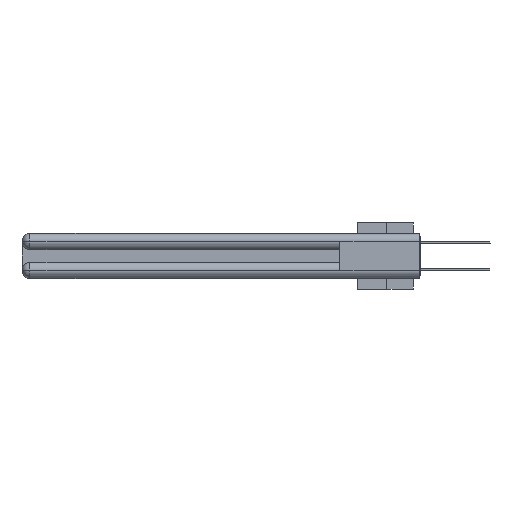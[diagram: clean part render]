
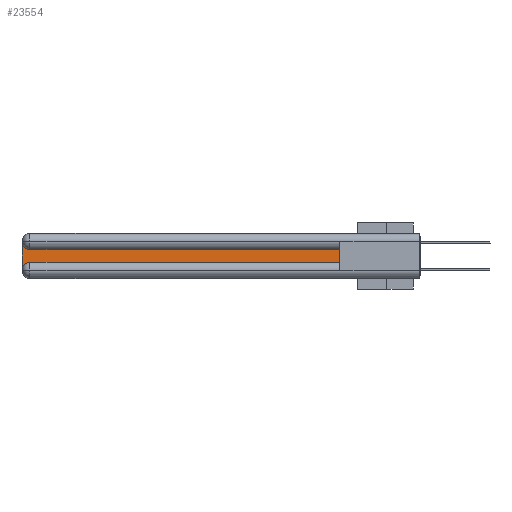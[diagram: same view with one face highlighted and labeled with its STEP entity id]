
A CAD part, left-side view. The second image highlights one B-rep face of the part: STEP entity #23554.
In plain terms, the highlighted planar face has unit normal (-1, 0, 0).
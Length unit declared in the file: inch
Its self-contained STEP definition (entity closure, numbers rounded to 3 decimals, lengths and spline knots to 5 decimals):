
#914 = CARTESIAN_POINT ( 'NONE',  ( 0.075, 2.94, -0.2775 ) ) ;
#1142 = DIRECTION ( 'NONE',  ( 1., 0., 0. ) ) ;
#2474 = VERTEX_POINT ( 'NONE', #17061 ) ;
#2644 = EDGE_CURVE ( 'NONE', #6175, #24458, #26580, .T. ) ;
#3265 = DIRECTION ( 'NONE',  ( 1., 0., 0. ) ) ;
#3273 = DIRECTION ( 'NONE',  ( 0., 0., -1. ) ) ;
#4350 = ORIENTED_EDGE ( 'NONE', *, *, #5753, .T. ) ;
#4694 = CARTESIAN_POINT ( 'NONE',  ( 0.075, 0.6, -0.1225 ) ) ;
#5704 = EDGE_CURVE ( 'NONE', #15519, #9257, #32199, .T. ) ;
#5753 = EDGE_CURVE ( 'NONE', #24458, #15519, #16304, .T. ) ;
#6175 = VERTEX_POINT ( 'NONE', #34233 ) ;
#7078 = EDGE_LOOP ( 'NONE', ( #9344, #14548, #9575, #26792, #8776, #4350 ) ) ;
#8245 = CARTESIAN_POINT ( 'NONE',  ( 0.075, 0.6, -0.2175 ) ) ;
#8471 = FACE_OUTER_BOUND ( 'NONE', #7078, .T. ) ;
#8776 = ORIENTED_EDGE ( 'NONE', *, *, #2644, .T. ) ;
#9257 = VERTEX_POINT ( 'NONE', #30815 ) ;
#9344 = ORIENTED_EDGE ( 'NONE', *, *, #5704, .T. ) ;
#9575 = ORIENTED_EDGE ( 'NONE', *, *, #25790, .T. ) ;
#10048 = DIRECTION ( 'NONE',  ( 0., -1., 0. ) ) ;
#10957 = CIRCLE ( 'NONE', #33094, 0.06 ) ;
#11924 = DIRECTION ( 'NONE',  ( 1., 0., 0. ) ) ;
#13236 = VECTOR ( 'NONE', #3273, 39.37008 ) ;
#14474 = LINE ( 'NONE', #16485, #13236 ) ;
#14548 = ORIENTED_EDGE ( 'NONE', *, *, #28262, .T. ) ;
#14812 = AXIS2_PLACEMENT_3D ( 'NONE', #914, #3265, #21833 ) ;
#14830 = VERTEX_POINT ( 'NONE', #31463 ) ;
#15070 = AXIS2_PLACEMENT_3D ( 'NONE', #19814, #1142, #19697 ) ;
#15337 = CIRCLE ( 'NONE', #14812, 0.06 ) ;
#15519 = VERTEX_POINT ( 'NONE', #4694 ) ;
#15888 = VECTOR ( 'NONE', #32841, 39.37008 ) ;
#16304 = LINE ( 'NONE', #19170, #15888 ) ;
#16485 = CARTESIAN_POINT ( 'NONE',  ( 0.075, 3., -0.2175 ) ) ;
#17061 = CARTESIAN_POINT ( 'NONE',  ( 0.075, 3., -0.2775 ) ) ;
#17626 = CARTESIAN_POINT ( 'NONE',  ( 0.075, 0.6, -0.2175 ) ) ;
#19170 = CARTESIAN_POINT ( 'NONE',  ( 0.075, 0.6, -0.2175 ) ) ;
#19697 = DIRECTION ( 'NONE',  ( 0., 0., -1. ) ) ;
#19814 = CARTESIAN_POINT ( 'NONE',  ( 0.075, 3., -0.1225 ) ) ;
#21360 = EDGE_CURVE ( 'NONE', #2474, #6175, #15337, .T. ) ;
#21542 = VECTOR ( 'NONE', #10048, 39.37008 ) ;
#21632 = CARTESIAN_POINT ( 'NONE',  ( 0.075, 0.6, -0.1225 ) ) ;
#21833 = DIRECTION ( 'NONE',  ( 0., 0., -1. ) ) ;
#23554 = ADVANCED_FACE ( 'NONE', ( #8471 ), #30578, .F. ) ;
#23834 = VECTOR ( 'NONE', #30043, 39.37008 ) ;
#24458 = VERTEX_POINT ( 'NONE', #8245 ) ;
#25581 = DIRECTION ( 'NONE',  ( 0., 0., -1. ) ) ;
#25790 = EDGE_CURVE ( 'NONE', #14830, #2474, #14474, .T. ) ;
#26580 = LINE ( 'NONE', #17626, #21542 ) ;
#26792 = ORIENTED_EDGE ( 'NONE', *, *, #21360, .T. ) ;
#28039 = CARTESIAN_POINT ( 'NONE',  ( 0.075, 2.94, -0.0625 ) ) ;
#28262 = EDGE_CURVE ( 'NONE', #9257, #14830, #10957, .T. ) ;
#30043 = DIRECTION ( 'NONE',  ( 0., 1., 0. ) ) ;
#30578 = PLANE ( 'NONE',  #15070 ) ;
#30815 = CARTESIAN_POINT ( 'NONE',  ( 0.075, 2.94, -0.1225 ) ) ;
#31463 = CARTESIAN_POINT ( 'NONE',  ( 0.075, 3., -0.0625 ) ) ;
#32199 = LINE ( 'NONE', #21632, #23834 ) ;
#32841 = DIRECTION ( 'NONE',  ( 0., 0., 1. ) ) ;
#33094 = AXIS2_PLACEMENT_3D ( 'NONE', #28039, #11924, #25581 ) ;
#34233 = CARTESIAN_POINT ( 'NONE',  ( 0.075, 2.94, -0.2175 ) ) ;
